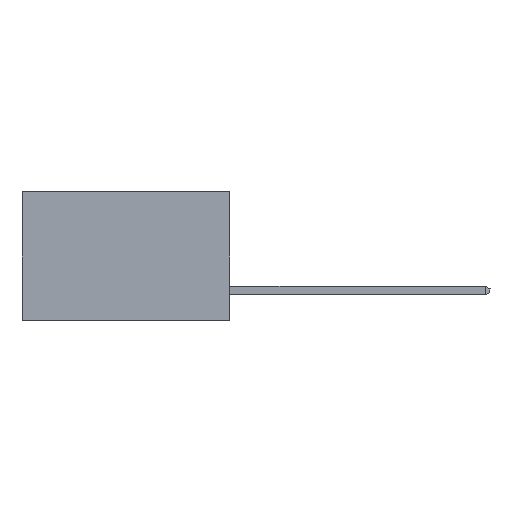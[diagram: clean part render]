
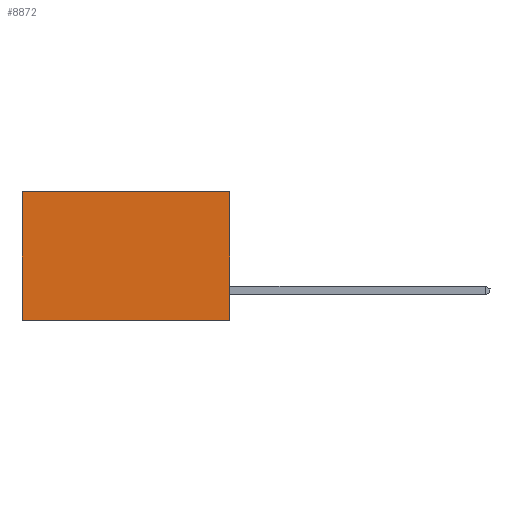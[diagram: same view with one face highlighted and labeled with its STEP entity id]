
A CAD part, left-side view. The second image highlights one B-rep face of the part: STEP entity #8872.
In plain terms, the highlighted planar face has unit normal (-1, 0, 0).
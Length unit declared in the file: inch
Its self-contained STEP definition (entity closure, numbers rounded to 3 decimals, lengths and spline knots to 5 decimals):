
#226 = DIRECTION ( 'NONE',  ( 0., 0., -1. ) ) ;
#304 = LINE ( 'NONE', #4480, #3988 ) ;
#482 = DIRECTION ( 'NONE',  ( 0., 1., 0. ) ) ;
#531 = LINE ( 'NONE', #4230, #2263 ) ;
#566 = LINE ( 'NONE', #6264, #7342 ) ;
#643 = VERTEX_POINT ( 'NONE', #5703 ) ;
#944 = CARTESIAN_POINT ( 'NONE',  ( 0.2615, 0.6, 0. ) ) ;
#1050 = EDGE_CURVE ( 'NONE', #3625, #643, #566, .T. ) ;
#1774 = ORIENTED_EDGE ( 'NONE', *, *, #3220, .T. ) ;
#1784 = ORIENTED_EDGE ( 'NONE', *, *, #1050, .F. ) ;
#1876 = DIRECTION ( 'NONE',  ( 0., 0., -1. ) ) ;
#1968 = FACE_OUTER_BOUND ( 'NONE', #3049, .T. ) ;
#2263 = VECTOR ( 'NONE', #482, 39.37008 ) ;
#3049 = EDGE_LOOP ( 'NONE', ( #3275, #1784, #7046, #1774 ) ) ;
#3220 = EDGE_CURVE ( 'NONE', #4076, #6552, #531, .T. ) ;
#3275 = ORIENTED_EDGE ( 'NONE', *, *, #9142, .T. ) ;
#3419 = CARTESIAN_POINT ( 'NONE',  ( 0.2615, 0., -0.37 ) ) ;
#3625 = VERTEX_POINT ( 'NONE', #6345 ) ;
#3772 = DIRECTION ( 'NONE',  ( 0., 0., -1. ) ) ;
#3988 = VECTOR ( 'NONE', #3772, 39.37008 ) ;
#4076 = VERTEX_POINT ( 'NONE', #4148 ) ;
#4148 = CARTESIAN_POINT ( 'NONE',  ( 0.2615, 0., 0. ) ) ;
#4230 = CARTESIAN_POINT ( 'NONE',  ( 0.2615, 0., 0. ) ) ;
#4480 = CARTESIAN_POINT ( 'NONE',  ( 0.2615, 0.6, -0.37 ) ) ;
#4675 = DIRECTION ( 'NONE',  ( 1., 0., 0. ) ) ;
#4784 = DIRECTION ( 'NONE',  ( 0., 1., 0. ) ) ;
#5490 = VECTOR ( 'NONE', #226, 39.37008 ) ;
#5703 = CARTESIAN_POINT ( 'NONE',  ( 0.2615, 0.6, -0.37 ) ) ;
#6264 = CARTESIAN_POINT ( 'NONE',  ( 0.2615, 0., -0.37 ) ) ;
#6345 = CARTESIAN_POINT ( 'NONE',  ( 0.2615, 0., -0.37 ) ) ;
#6552 = VERTEX_POINT ( 'NONE', #944 ) ;
#6716 = LINE ( 'NONE', #7529, #5490 ) ;
#6998 = PLANE ( 'NONE',  #8220 ) ;
#7046 = ORIENTED_EDGE ( 'NONE', *, *, #8261, .F. ) ;
#7342 = VECTOR ( 'NONE', #4784, 39.37008 ) ;
#7529 = CARTESIAN_POINT ( 'NONE',  ( 0.2615, 0., -0.37 ) ) ;
#8220 = AXIS2_PLACEMENT_3D ( 'NONE', #3419, #4675, #1876 ) ;
#8261 = EDGE_CURVE ( 'NONE', #4076, #3625, #6716, .T. ) ;
#8872 = ADVANCED_FACE ( 'NONE', ( #1968 ), #6998, .F. ) ;
#9142 = EDGE_CURVE ( 'NONE', #6552, #643, #304, .T. ) ;
